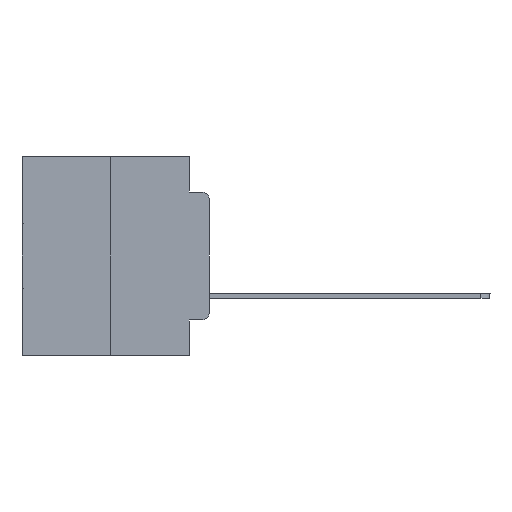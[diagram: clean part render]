
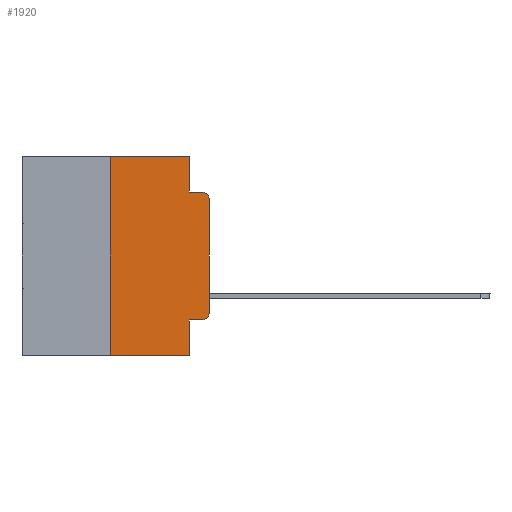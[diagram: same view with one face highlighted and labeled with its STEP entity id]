
A CAD part, left-side view. The second image highlights one B-rep face of the part: STEP entity #1920.
In plain terms, the highlighted planar face has unit normal (-1, 0, 0).
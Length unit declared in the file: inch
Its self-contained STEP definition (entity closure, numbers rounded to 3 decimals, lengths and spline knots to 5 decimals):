
#2 = CIRCLE ( 'NONE', #19839, 0.02 ) ;
#216 = FACE_OUTER_BOUND ( 'NONE', #13977, .T. ) ;
#412 = ORIENTED_EDGE ( 'NONE', *, *, #4032, .F. ) ;
#986 = CARTESIAN_POINT ( 'NONE',  ( 0., 0.473, -0.5 ) ) ;
#1061 = CARTESIAN_POINT ( 'NONE',  ( 0., 0.25, 0. ) ) ;
#1589 = AXIS2_PLACEMENT_3D ( 'NONE', #13375, #6729, #23288 ) ;
#1631 = LINE ( 'NONE', #20826, #7835 ) ;
#1920 = ADVANCED_FACE ( 'NONE', ( #216 ), #15632, .F. ) ;
#1968 = ORIENTED_EDGE ( 'NONE', *, *, #4186, .F. ) ;
#3703 = CARTESIAN_POINT ( 'NONE',  ( 0., 0.051, -0.0885 ) ) ;
#4032 = EDGE_CURVE ( 'NONE', #21224, #23912, #16843, .T. ) ;
#4186 = EDGE_CURVE ( 'NONE', #16681, #21224, #21908, .T. ) ;
#4365 = VECTOR ( 'NONE', #12252, 39.37008 ) ;
#4436 = VERTEX_POINT ( 'NONE', #25542 ) ;
#4636 = CARTESIAN_POINT ( 'NONE',  ( 0., 0.051, -0.4115 ) ) ;
#4832 = CARTESIAN_POINT ( 'NONE',  ( 0., 0., -0.3915 ) ) ;
#5189 = VECTOR ( 'NONE', #14467, 39.37008 ) ;
#5506 = LINE ( 'NONE', #986, #23844 ) ;
#5830 = EDGE_CURVE ( 'NONE', #11081, #23912, #18721, .T. ) ;
#6018 = LINE ( 'NONE', #21384, #4365 ) ;
#6522 = CARTESIAN_POINT ( 'NONE',  ( 0., 0.051, -0.4115 ) ) ;
#6583 = VERTEX_POINT ( 'NONE', #26118 ) ;
#6729 = DIRECTION ( 'NONE',  ( 1., 0., 0. ) ) ;
#6841 = ORIENTED_EDGE ( 'NONE', *, *, #19938, .F. ) ;
#7736 = DIRECTION ( 'NONE',  ( 0., -1., 0. ) ) ;
#7835 = VECTOR ( 'NONE', #7736, 39.37008 ) ;
#8106 = DIRECTION ( 'NONE',  ( -1., 0., 0. ) ) ;
#8695 = CARTESIAN_POINT ( 'NONE',  ( 0., 0.051, 0. ) ) ;
#9574 = ORIENTED_EDGE ( 'NONE', *, *, #5830, .T. ) ;
#9669 = EDGE_CURVE ( 'NONE', #11260, #26260, #24914, .T. ) ;
#9742 = ORIENTED_EDGE ( 'NONE', *, *, #24937, .T. ) ;
#9923 = VECTOR ( 'NONE', #13030, 39.37008 ) ;
#10501 = EDGE_CURVE ( 'NONE', #6583, #24287, #2, .T. ) ;
#10810 = VECTOR ( 'NONE', #26615, 39.37008 ) ;
#11081 = VERTEX_POINT ( 'NONE', #19672 ) ;
#11260 = VERTEX_POINT ( 'NONE', #24614 ) ;
#11621 = ORIENTED_EDGE ( 'NONE', *, *, #15355, .T. ) ;
#12252 = DIRECTION ( 'NONE',  ( 0., 0., 1. ) ) ;
#13030 = DIRECTION ( 'NONE',  ( 0., -1., 0. ) ) ;
#13375 = CARTESIAN_POINT ( 'NONE',  ( 0., 0.473, 0. ) ) ;
#13456 = CARTESIAN_POINT ( 'NONE',  ( 0., 0.051, 0. ) ) ;
#13734 = DIRECTION ( 'NONE',  ( -1., 0., 0. ) ) ;
#13977 = EDGE_LOOP ( 'NONE', ( #9742, #9574, #412, #1968, #6841, #25018, #11621, #25947, #24281, #14549 ) ) ;
#14206 = CARTESIAN_POINT ( 'NONE',  ( 0., 0.02, -0.1085 ) ) ;
#14467 = DIRECTION ( 'NONE',  ( 0., -1., 0. ) ) ;
#14549 = ORIENTED_EDGE ( 'NONE', *, *, #10501, .T. ) ;
#15355 = EDGE_CURVE ( 'NONE', #11260, #4436, #5506, .T. ) ;
#15496 = VECTOR ( 'NONE', #27875, 39.37008 ) ;
#15607 = VECTOR ( 'NONE', #24158, 39.37008 ) ;
#15632 = PLANE ( 'NONE',  #1589 ) ;
#15972 = DIRECTION ( 'NONE',  ( 0., -1., 0. ) ) ;
#16681 = VERTEX_POINT ( 'NONE', #20076 ) ;
#16843 = LINE ( 'NONE', #3703, #5189 ) ;
#17250 = LINE ( 'NONE', #6522, #9923 ) ;
#18409 = DIRECTION ( 'NONE',  ( 0., 0., -1. ) ) ;
#18721 = CIRCLE ( 'NONE', #23742, 0.02 ) ;
#19357 = CARTESIAN_POINT ( 'NONE',  ( 0., 0.25, 0. ) ) ;
#19672 = CARTESIAN_POINT ( 'NONE',  ( 0., 0., -0.1085 ) ) ;
#19839 = AXIS2_PLACEMENT_3D ( 'NONE', #24434, #13734, #22329 ) ;
#19938 = EDGE_CURVE ( 'NONE', #26260, #16681, #1631, .T. ) ;
#19952 = CARTESIAN_POINT ( 'NONE',  ( 0., 0.02, -0.0885 ) ) ;
#20076 = CARTESIAN_POINT ( 'NONE',  ( 0., 0.051, 0. ) ) ;
#20826 = CARTESIAN_POINT ( 'NONE',  ( 0., 0.473, 0. ) ) ;
#21224 = VERTEX_POINT ( 'NONE', #26052 ) ;
#21299 = EDGE_CURVE ( 'NONE', #26747, #4436, #21389, .T. ) ;
#21384 = CARTESIAN_POINT ( 'NONE',  ( 0., 0., 0. ) ) ;
#21389 = LINE ( 'NONE', #8695, #15496 ) ;
#21908 = LINE ( 'NONE', #13456, #15607 ) ;
#22329 = DIRECTION ( 'NONE',  ( 0., 0., -1. ) ) ;
#23288 = DIRECTION ( 'NONE',  ( 0., 0., -1. ) ) ;
#23742 = AXIS2_PLACEMENT_3D ( 'NONE', #14206, #8106, #18409 ) ;
#23844 = VECTOR ( 'NONE', #15972, 39.37008 ) ;
#23912 = VERTEX_POINT ( 'NONE', #19952 ) ;
#24158 = DIRECTION ( 'NONE',  ( 0., 0., -1. ) ) ;
#24281 = ORIENTED_EDGE ( 'NONE', *, *, #26303, .T. ) ;
#24287 = VERTEX_POINT ( 'NONE', #4832 ) ;
#24434 = CARTESIAN_POINT ( 'NONE',  ( 0., 0.02, -0.3915 ) ) ;
#24614 = CARTESIAN_POINT ( 'NONE',  ( 0., 0.25, -0.5 ) ) ;
#24914 = LINE ( 'NONE', #1061, #10810 ) ;
#24937 = EDGE_CURVE ( 'NONE', #24287, #11081, #6018, .T. ) ;
#25018 = ORIENTED_EDGE ( 'NONE', *, *, #9669, .F. ) ;
#25542 = CARTESIAN_POINT ( 'NONE',  ( 0., 0.051, -0.5 ) ) ;
#25947 = ORIENTED_EDGE ( 'NONE', *, *, #21299, .F. ) ;
#26052 = CARTESIAN_POINT ( 'NONE',  ( 0., 0.051, -0.0885 ) ) ;
#26118 = CARTESIAN_POINT ( 'NONE',  ( 0., 0.02, -0.4115 ) ) ;
#26260 = VERTEX_POINT ( 'NONE', #19357 ) ;
#26303 = EDGE_CURVE ( 'NONE', #26747, #6583, #17250, .T. ) ;
#26615 = DIRECTION ( 'NONE',  ( 0., 0., 1. ) ) ;
#26747 = VERTEX_POINT ( 'NONE', #4636 ) ;
#27875 = DIRECTION ( 'NONE',  ( 0., 0., -1. ) ) ;
